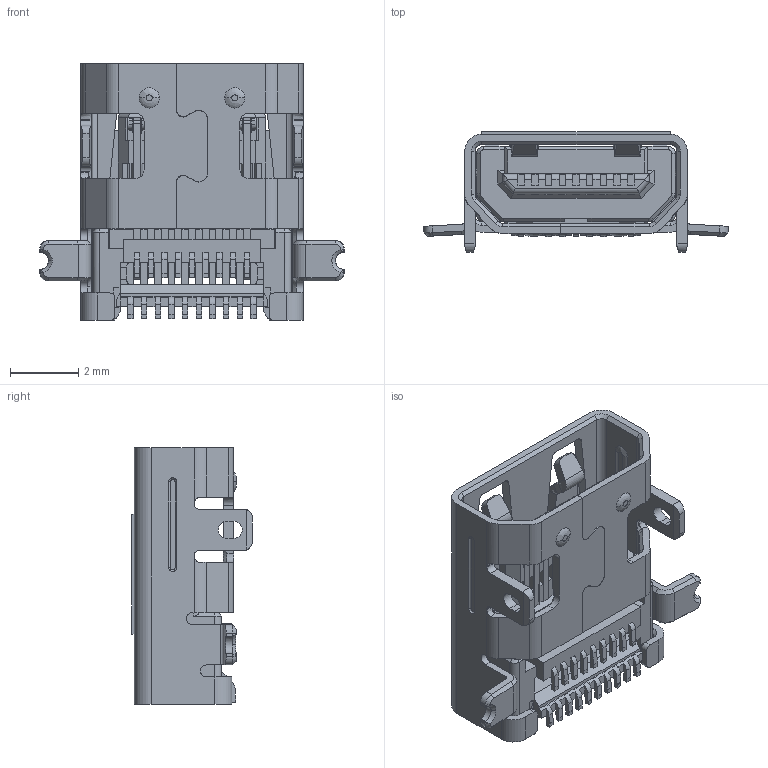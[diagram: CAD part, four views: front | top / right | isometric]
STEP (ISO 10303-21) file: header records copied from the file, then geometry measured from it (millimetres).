
FILE_DESCRIPTION (( 'STEP AP214' ), '1' );
FILE_NAME ('694H319-169-211.STEP', '2021-01-13T18:51:16', ( '' ), ( '' ), 'SwSTEP 2.0', 'SolidWorks 2020', '' );
FILE_SCHEMA (( 'AUTOMOTIVE_DESIGN' ));
Length unit declared in the file: millimetre
Products named in the file (4): Shell 694H319-X69-211; Tape 694H319-X69-211; Insulator 694H319-X69-211; 694H319-169-211
Assembly tree (3 placements, depth 2):
  694H319-169-211
    Insulator 694H319-X69-211
    Shell 694H319-X69-211
    Tape 694H319-X69-211
Bounding box: 8.9 x 3.53 x 7.5 mm (x, y, z)
Volume: 62.3 mm3; surface area: 459.3 mm2
Topology: 3 solids, 3 shells, 1453 faces, 4216 edges, 2682 vertices
Faces by surface type: plane 1130, cylinder 217, cone 70, bspline 36
Entity records: 60351 total; most frequent: CARTESIAN_POINT 11908, ORIENTED_EDGE 8414, DIRECTION 6681, EDGE_CURVE 4207, LINE 3239, VECTOR 3239, VERTEX_POINT 2682, AXIS2_PLACEMENT_3D 1721
